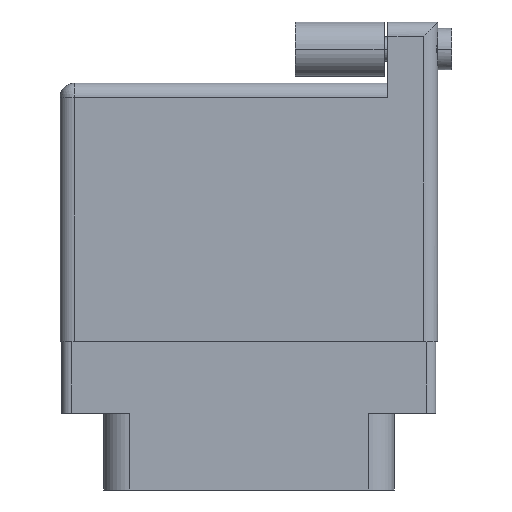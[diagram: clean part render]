
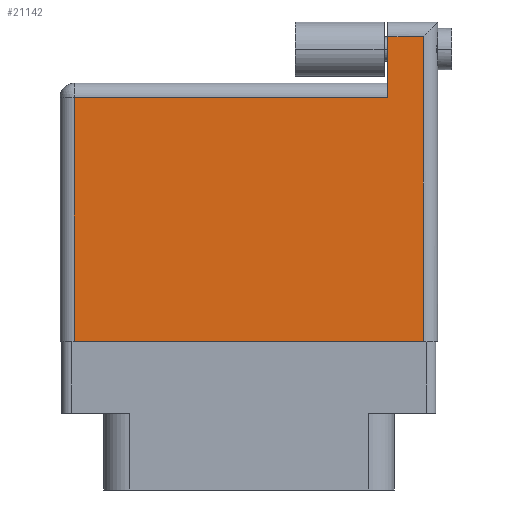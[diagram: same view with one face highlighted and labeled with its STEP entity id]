
A CAD part, front view. The second image highlights one B-rep face of the part: STEP entity #21142.
In plain terms, the highlighted face is planar.
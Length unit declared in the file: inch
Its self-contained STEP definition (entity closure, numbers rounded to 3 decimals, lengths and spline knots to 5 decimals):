
#25 = CARTESIAN_POINT ( 'NONE',  ( 1.275, 0., 0. ) ) ;
#1446 = CARTESIAN_POINT ( 'NONE',  ( 0.05, 0.856, 0. ) ) ;
#1539 = ORIENTED_EDGE ( 'NONE', *, *, #24700, .T. ) ;
#1584 = VECTOR ( 'NONE', #13626, 39.37008 ) ;
#2268 = ORIENTED_EDGE ( 'NONE', *, *, #9387, .T. ) ;
#2984 = VERTEX_POINT ( 'NONE', #16717 ) ;
#3013 = CARTESIAN_POINT ( 'NONE',  ( 0., 0.906, 0. ) ) ;
#3234 = EDGE_CURVE ( 'NONE', #8765, #7555, #8527, .T. ) ;
#4238 = DIRECTION ( 'NONE',  ( 0., 1., 0. ) ) ;
#4263 = LINE ( 'NONE', #18555, #7021 ) ;
#4284 = CARTESIAN_POINT ( 'NONE',  ( 1.15, 1.07, 0. ) ) ;
#4541 = EDGE_CURVE ( 'NONE', #2984, #18037, #11960, .T. ) ;
#4611 = LINE ( 'NONE', #21297, #14257 ) ;
#5747 = CARTESIAN_POINT ( 'NONE',  ( 1.275, 1.12, 0. ) ) ;
#6901 = VECTOR ( 'NONE', #4238, 39.37008 ) ;
#6993 = VERTEX_POINT ( 'NONE', #4284 ) ;
#7021 = VECTOR ( 'NONE', #10414, 39.37008 ) ;
#7096 = DIRECTION ( 'NONE',  ( 0., -1., 0. ) ) ;
#7555 = VERTEX_POINT ( 'NONE', #10376 ) ;
#7987 = LINE ( 'NONE', #26131, #16700 ) ;
#8527 = LINE ( 'NONE', #5747, #6901 ) ;
#8579 = ORIENTED_EDGE ( 'NONE', *, *, #3234, .T. ) ;
#8765 = VERTEX_POINT ( 'NONE', #25 ) ;
#9387 = EDGE_CURVE ( 'NONE', #18037, #19852, #7987, .T. ) ;
#9783 = EDGE_CURVE ( 'NONE', #7555, #6993, #4611, .T. ) ;
#10376 = CARTESIAN_POINT ( 'NONE',  ( 1.275, 1.07, 0. ) ) ;
#10414 = DIRECTION ( 'NONE',  ( 1., 0., 0. ) ) ;
#11010 = ORIENTED_EDGE ( 'NONE', *, *, #9783, .T. ) ;
#11960 = LINE ( 'NONE', #26248, #21008 ) ;
#12611 = AXIS2_PLACEMENT_3D ( 'NONE', #3013, #15446, #19302 ) ;
#13626 = DIRECTION ( 'NONE',  ( 0., -1., 0. ) ) ;
#14257 = VECTOR ( 'NONE', #19147, 39.37008 ) ;
#15184 = FACE_OUTER_BOUND ( 'NONE', #25797, .T. ) ;
#15446 = DIRECTION ( 'NONE',  ( 0., 0., -1. ) ) ;
#15969 = DIRECTION ( 'NONE',  ( -1., 0., 0. ) ) ;
#16700 = VECTOR ( 'NONE', #7096, 39.37008 ) ;
#16717 = CARTESIAN_POINT ( 'NONE',  ( 1.15, 0.856, 0. ) ) ;
#17490 = LINE ( 'NONE', #23660, #1584 ) ;
#18037 = VERTEX_POINT ( 'NONE', #1446 ) ;
#18555 = CARTESIAN_POINT ( 'NONE',  ( 0., 0., 0. ) ) ;
#19147 = DIRECTION ( 'NONE',  ( -1., 0., 0. ) ) ;
#19215 = EDGE_CURVE ( 'NONE', #19852, #8765, #4263, .T. ) ;
#19302 = DIRECTION ( 'NONE',  ( -1., 0., 0. ) ) ;
#19852 = VERTEX_POINT ( 'NONE', #23720 ) ;
#21008 = VECTOR ( 'NONE', #15969, 39.37008 ) ;
#21142 = ADVANCED_FACE ( 'NONE', ( #15184 ), #23331, .F. ) ;
#21297 = CARTESIAN_POINT ( 'NONE',  ( 0., 1.07, 0. ) ) ;
#21643 = ORIENTED_EDGE ( 'NONE', *, *, #4541, .T. ) ;
#23331 = PLANE ( 'NONE',  #12611 ) ;
#23660 = CARTESIAN_POINT ( 'NONE',  ( 1.15, 1.12, 0. ) ) ;
#23720 = CARTESIAN_POINT ( 'NONE',  ( 0.05, 0., 0. ) ) ;
#24700 = EDGE_CURVE ( 'NONE', #6993, #2984, #17490, .T. ) ;
#24710 = ORIENTED_EDGE ( 'NONE', *, *, #19215, .T. ) ;
#25797 = EDGE_LOOP ( 'NONE', ( #24710, #8579, #11010, #1539, #21643, #2268 ) ) ;
#26131 = CARTESIAN_POINT ( 'NONE',  ( 0.05, 0., 0. ) ) ;
#26248 = CARTESIAN_POINT ( 'NONE',  ( 0., 0.856, 0. ) ) ;
